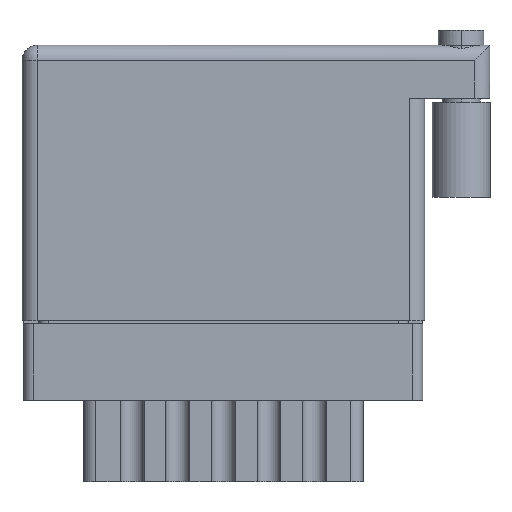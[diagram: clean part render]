
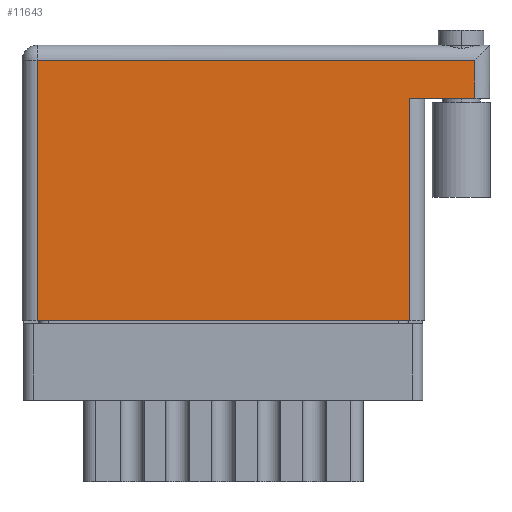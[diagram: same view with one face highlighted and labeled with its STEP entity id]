
A CAD part, front view. The second image highlights one B-rep face of the part: STEP entity #11643.
In plain terms, the highlighted face is planar.
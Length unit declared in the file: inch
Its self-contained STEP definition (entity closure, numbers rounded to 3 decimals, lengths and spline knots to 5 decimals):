
#1285 = ORIENTED_EDGE ( 'NONE', *, *, #2771, .F. ) ;
#2168 = CARTESIAN_POINT ( 'NONE',  ( 0., 0.906, 0. ) ) ;
#2404 = CARTESIAN_POINT ( 'NONE',  ( 1.275, 0.731, 0. ) ) ;
#2602 = CARTESIAN_POINT ( 'NONE',  ( 1.539, 0.731, 0. ) ) ;
#2771 = EDGE_CURVE ( 'NONE', #12134, #6381, #14302, .T. ) ;
#2934 = EDGE_CURVE ( 'NONE', #13876, #6381, #11035, .T. ) ;
#4710 = EDGE_CURVE ( 'NONE', #9188, #22749, #17038, .T. ) ;
#4878 = DIRECTION ( 'NONE',  ( 0., -1., 0. ) ) ;
#4891 = EDGE_CURVE ( 'NONE', #12134, #9188, #10386, .T. ) ;
#6381 = VERTEX_POINT ( 'NONE', #19014 ) ;
#7781 = CARTESIAN_POINT ( 'NONE',  ( 1.489, 0.906, 0. ) ) ;
#8303 = CARTESIAN_POINT ( 'NONE',  ( 1.275, 0., 0. ) ) ;
#9188 = VERTEX_POINT ( 'NONE', #14930 ) ;
#9268 = DIRECTION ( 'NONE',  ( 0., 0., -1. ) ) ;
#9420 = DIRECTION ( 'NONE',  ( -1., 0., 0. ) ) ;
#9533 = CARTESIAN_POINT ( 'NONE',  ( 1.489, 0.731, 0. ) ) ;
#9562 = LINE ( 'NONE', #11397, #14862 ) ;
#10386 = LINE ( 'NONE', #7781, #22409 ) ;
#10852 = ORIENTED_EDGE ( 'NONE', *, *, #16401, .T. ) ;
#11035 = LINE ( 'NONE', #2404, #21274 ) ;
#11077 = VECTOR ( 'NONE', #19490, 39.37008 ) ;
#11200 = EDGE_CURVE ( 'NONE', #22749, #16439, #28765, .T. ) ;
#11397 = CARTESIAN_POINT ( 'NONE',  ( 0., 0., 0. ) ) ;
#11643 = ADVANCED_FACE ( 'NONE', ( #24991 ), #16358, .F. ) ;
#11977 = DIRECTION ( 'NONE',  ( -1., 0., 0. ) ) ;
#12134 = VERTEX_POINT ( 'NONE', #9533 ) ;
#13868 = DIRECTION ( 'NONE',  ( 1., 0., 0. ) ) ;
#13876 = VERTEX_POINT ( 'NONE', #8303 ) ;
#14302 = LINE ( 'NONE', #2602, #28145 ) ;
#14586 = CARTESIAN_POINT ( 'NONE',  ( 0.05, 0., 0. ) ) ;
#14862 = VECTOR ( 'NONE', #13868, 39.37008 ) ;
#14930 = CARTESIAN_POINT ( 'NONE',  ( 1.489, 0.856, 0. ) ) ;
#15470 = CARTESIAN_POINT ( 'NONE',  ( 0.05, 0.856, 0. ) ) ;
#15979 = DIRECTION ( 'NONE',  ( 0., 1., 0. ) ) ;
#16308 = ORIENTED_EDGE ( 'NONE', *, *, #11200, .T. ) ;
#16358 = PLANE ( 'NONE',  #28645 ) ;
#16401 = EDGE_CURVE ( 'NONE', #16439, #13876, #9562, .T. ) ;
#16439 = VERTEX_POINT ( 'NONE', #25586 ) ;
#16592 = EDGE_LOOP ( 'NONE', ( #10852, #17494, #1285, #26289, #19065, #16308 ) ) ;
#17038 = LINE ( 'NONE', #26426, #11077 ) ;
#17494 = ORIENTED_EDGE ( 'NONE', *, *, #2934, .T. ) ;
#19014 = CARTESIAN_POINT ( 'NONE',  ( 1.275, 0.731, 0. ) ) ;
#19065 = ORIENTED_EDGE ( 'NONE', *, *, #4710, .T. ) ;
#19490 = DIRECTION ( 'NONE',  ( -1., 0., 0. ) ) ;
#19800 = DIRECTION ( 'NONE',  ( 0., 1., 0. ) ) ;
#19828 = VECTOR ( 'NONE', #4878, 39.37008 ) ;
#21274 = VECTOR ( 'NONE', #15979, 39.37008 ) ;
#22409 = VECTOR ( 'NONE', #19800, 39.37008 ) ;
#22749 = VERTEX_POINT ( 'NONE', #15470 ) ;
#24991 = FACE_OUTER_BOUND ( 'NONE', #16592, .T. ) ;
#25586 = CARTESIAN_POINT ( 'NONE',  ( 0.05, 0., 0. ) ) ;
#26289 = ORIENTED_EDGE ( 'NONE', *, *, #4891, .T. ) ;
#26426 = CARTESIAN_POINT ( 'NONE',  ( 0., 0.856, 0. ) ) ;
#28145 = VECTOR ( 'NONE', #11977, 39.37008 ) ;
#28645 = AXIS2_PLACEMENT_3D ( 'NONE', #2168, #9268, #9420 ) ;
#28765 = LINE ( 'NONE', #14586, #19828 ) ;
